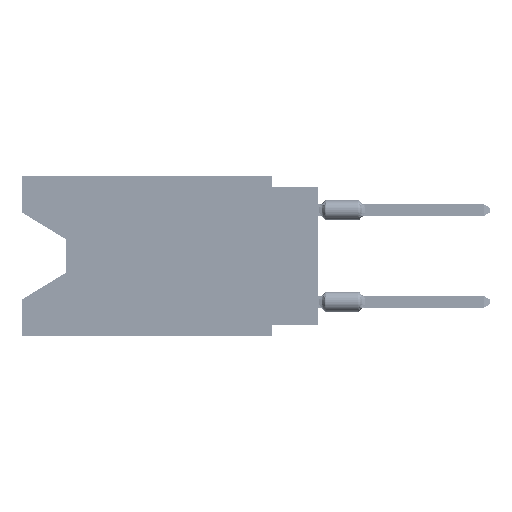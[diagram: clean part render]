
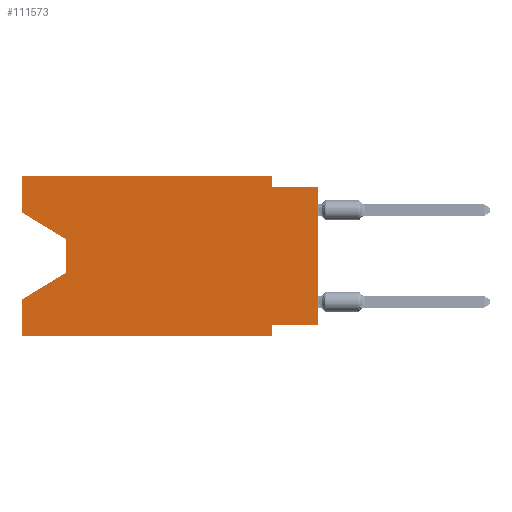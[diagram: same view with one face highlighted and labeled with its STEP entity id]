
A CAD part, left-side view. The second image highlights one B-rep face of the part: STEP entity #111573.
In plain terms, the highlighted planar face has unit normal (-1, 0, 0).
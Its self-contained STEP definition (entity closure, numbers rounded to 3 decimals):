
#874 = DIRECTION ( 'NONE',  ( 0., 0., 1. ) ) ;
#950 = CARTESIAN_POINT ( 'NONE',  ( 0., 16.383, 0. ) ) ;
#1148 = VERTEX_POINT ( 'NONE', #42550 ) ;
#1675 = CARTESIAN_POINT ( 'NONE',  ( 0., 16.383, -2.038 ) ) ;
#4201 = CARTESIAN_POINT ( 'NONE',  ( 0., 0., -8.255 ) ) ;
#5272 = ORIENTED_EDGE ( 'NONE', *, *, #76750, .T. ) ;
#5719 = VECTOR ( 'NONE', #119918, 1000. ) ;
#7027 = EDGE_CURVE ( 'NONE', #1148, #25110, #29135, .T. ) ;
#7135 = ORIENTED_EDGE ( 'NONE', *, *, #63450, .F. ) ;
#9229 = AXIS2_PLACEMENT_3D ( 'NONE', #62400, #100708, #73324 ) ;
#11121 = CARTESIAN_POINT ( 'NONE',  ( 0., 2.54, -8.89 ) ) ;
#11260 = VECTOR ( 'NONE', #66752, 1000. ) ;
#11757 = ORIENTED_EDGE ( 'NONE', *, *, #52640, .F. ) ;
#14293 = ORIENTED_EDGE ( 'NONE', *, *, #109921, .T. ) ;
#14348 = VERTEX_POINT ( 'NONE', #950 ) ;
#14416 = CARTESIAN_POINT ( 'NONE',  ( 0., 13.97, -5.385 ) ) ;
#14577 = CARTESIAN_POINT ( 'NONE',  ( 0., 13.97, -3.505 ) ) ;
#15111 = CARTESIAN_POINT ( 'NONE',  ( 0., 13.97, -3.505 ) ) ;
#17755 = DIRECTION ( 'NONE',  ( 0., 0., 1. ) ) ;
#20256 = VERTEX_POINT ( 'NONE', #97292 ) ;
#24397 = CARTESIAN_POINT ( 'NONE',  ( 0., 16.383, 0. ) ) ;
#24576 = CARTESIAN_POINT ( 'NONE',  ( 0., 0., 0. ) ) ;
#25110 = VERTEX_POINT ( 'NONE', #11121 ) ;
#28257 = CARTESIAN_POINT ( 'NONE',  ( 0., 2.54, 0. ) ) ;
#28690 = DIRECTION ( 'NONE',  ( 0., -1., 0. ) ) ;
#28850 = CARTESIAN_POINT ( 'NONE',  ( 0., 16.383, 0. ) ) ;
#29135 = LINE ( 'NONE', #48588, #73090 ) ;
#29472 = EDGE_CURVE ( 'NONE', #20256, #25110, #113002, .T. ) ;
#30509 = ORIENTED_EDGE ( 'NONE', *, *, #69261, .F. ) ;
#31690 = ORIENTED_EDGE ( 'NONE', *, *, #47293, .F. ) ;
#31770 = CARTESIAN_POINT ( 'NONE',  ( 0., 16.383, -2.038 ) ) ;
#32011 = VERTEX_POINT ( 'NONE', #31770 ) ;
#33110 = LINE ( 'NONE', #24576, #104594 ) ;
#35797 = LINE ( 'NONE', #83243, #68841 ) ;
#35985 = LINE ( 'NONE', #101091, #87800 ) ;
#37369 = LINE ( 'NONE', #28850, #60421 ) ;
#41198 = EDGE_CURVE ( 'NONE', #14348, #94106, #70622, .T. ) ;
#42550 = CARTESIAN_POINT ( 'NONE',  ( 0., 2.54, -8.255 ) ) ;
#42722 = ORIENTED_EDGE ( 'NONE', *, *, #57323, .T. ) ;
#43103 = ORIENTED_EDGE ( 'NONE', *, *, #29472, .T. ) ;
#45715 = CARTESIAN_POINT ( 'NONE',  ( 0., 0., -0.635 ) ) ;
#45721 = CARTESIAN_POINT ( 'NONE',  ( 0., 13.97, -5.385 ) ) ;
#46137 = DIRECTION ( 'NONE',  ( 0., 0., -1. ) ) ;
#46704 = CARTESIAN_POINT ( 'NONE',  ( 0., 16.383, -8.89 ) ) ;
#47293 = EDGE_CURVE ( 'NONE', #109752, #1148, #63441, .T. ) ;
#48588 = CARTESIAN_POINT ( 'NONE',  ( 0., 2.54, -8.89 ) ) ;
#50520 = ORIENTED_EDGE ( 'NONE', *, *, #78127, .F. ) ;
#52358 = DIRECTION ( 'NONE',  ( 0., -1., 0. ) ) ;
#52568 = CARTESIAN_POINT ( 'NONE',  ( 0., 0., -0.635 ) ) ;
#52640 = EDGE_CURVE ( 'NONE', #32011, #14348, #37369, .T. ) ;
#53982 = EDGE_LOOP ( 'NONE', ( #14293, #42722, #5272, #7135, #43103, #100615, #31690, #61997, #50520, #30509, #119016, #11757 ) ) ;
#54335 = DIRECTION ( 'NONE',  ( 0., 1., 0. ) ) ;
#55523 = CARTESIAN_POINT ( 'NONE',  ( 0., 0., -8.255 ) ) ;
#56767 = CARTESIAN_POINT ( 'NONE',  ( 0., 2.54, -0.635 ) ) ;
#57323 = EDGE_CURVE ( 'NONE', #87203, #86443, #61915, .T. ) ;
#57604 = LINE ( 'NONE', #1675, #11260 ) ;
#59279 = DIRECTION ( 'NONE',  ( 0., 0., 1. ) ) ;
#60421 = VECTOR ( 'NONE', #874, 1000. ) ;
#61915 = LINE ( 'NONE', #15111, #65668 ) ;
#61917 = VECTOR ( 'NONE', #28690, 1000. ) ;
#61997 = ORIENTED_EDGE ( 'NONE', *, *, #111769, .T. ) ;
#62400 = CARTESIAN_POINT ( 'NONE',  ( 0., 16.383, 0. ) ) ;
#63370 = LINE ( 'NONE', #45721, #5719 ) ;
#63441 = LINE ( 'NONE', #55523, #94174 ) ;
#63450 = EDGE_CURVE ( 'NONE', #20256, #120114, #35985, .T. ) ;
#63584 = PLANE ( 'NONE',  #9229 ) ;
#64801 = FACE_OUTER_BOUND ( 'NONE', #53982, .T. ) ;
#65668 = VECTOR ( 'NONE', #118468, 1000. ) ;
#66752 = DIRECTION ( 'NONE',  ( 0., -0.855, -0.519 ) ) ;
#66777 = DIRECTION ( 'NONE',  ( 0., -1., 0. ) ) ;
#68841 = VECTOR ( 'NONE', #111213, 1000. ) ;
#69261 = EDGE_CURVE ( 'NONE', #94106, #105270, #35797, .T. ) ;
#70622 = LINE ( 'NONE', #24397, #73959 ) ;
#73090 = VECTOR ( 'NONE', #46137, 1000. ) ;
#73324 = DIRECTION ( 'NONE',  ( 0., 0., -1. ) ) ;
#73959 = VECTOR ( 'NONE', #52358, 1000. ) ;
#76750 = EDGE_CURVE ( 'NONE', #86443, #120114, #63370, .T. ) ;
#78127 = EDGE_CURVE ( 'NONE', #105270, #113159, #92543, .T. ) ;
#83243 = CARTESIAN_POINT ( 'NONE',  ( 0., 2.54, 0. ) ) ;
#86443 = VERTEX_POINT ( 'NONE', #14416 ) ;
#87203 = VERTEX_POINT ( 'NONE', #14577 ) ;
#87800 = VECTOR ( 'NONE', #17755, 1000. ) ;
#92543 = LINE ( 'NONE', #45715, #61917 ) ;
#94106 = VERTEX_POINT ( 'NONE', #28257 ) ;
#94174 = VECTOR ( 'NONE', #54335, 1000. ) ;
#97292 = CARTESIAN_POINT ( 'NONE',  ( 0., 16.383, -8.89 ) ) ;
#100615 = ORIENTED_EDGE ( 'NONE', *, *, #7027, .F. ) ;
#100708 = DIRECTION ( 'NONE',  ( 1., 0., 0. ) ) ;
#101091 = CARTESIAN_POINT ( 'NONE',  ( 0., 16.383, 0. ) ) ;
#104594 = VECTOR ( 'NONE', #59279, 1000. ) ;
#105270 = VERTEX_POINT ( 'NONE', #56767 ) ;
#109752 = VERTEX_POINT ( 'NONE', #4201 ) ;
#109921 = EDGE_CURVE ( 'NONE', #32011, #87203, #57604, .T. ) ;
#111213 = DIRECTION ( 'NONE',  ( 0., 0., -1. ) ) ;
#111573 = ADVANCED_FACE ( 'NONE', ( #64801 ), #63584, .F. ) ;
#111769 = EDGE_CURVE ( 'NONE', #109752, #113159, #33110, .T. ) ;
#112842 = CARTESIAN_POINT ( 'NONE',  ( 0., 16.383, -6.852 ) ) ;
#113002 = LINE ( 'NONE', #46704, #117057 ) ;
#113159 = VERTEX_POINT ( 'NONE', #52568 ) ;
#117057 = VECTOR ( 'NONE', #66777, 1000. ) ;
#118468 = DIRECTION ( 'NONE',  ( 0., 0., -1. ) ) ;
#119016 = ORIENTED_EDGE ( 'NONE', *, *, #41198, .F. ) ;
#119918 = DIRECTION ( 'NONE',  ( 0., 0.855, -0.519 ) ) ;
#120114 = VERTEX_POINT ( 'NONE', #112842 ) ;
